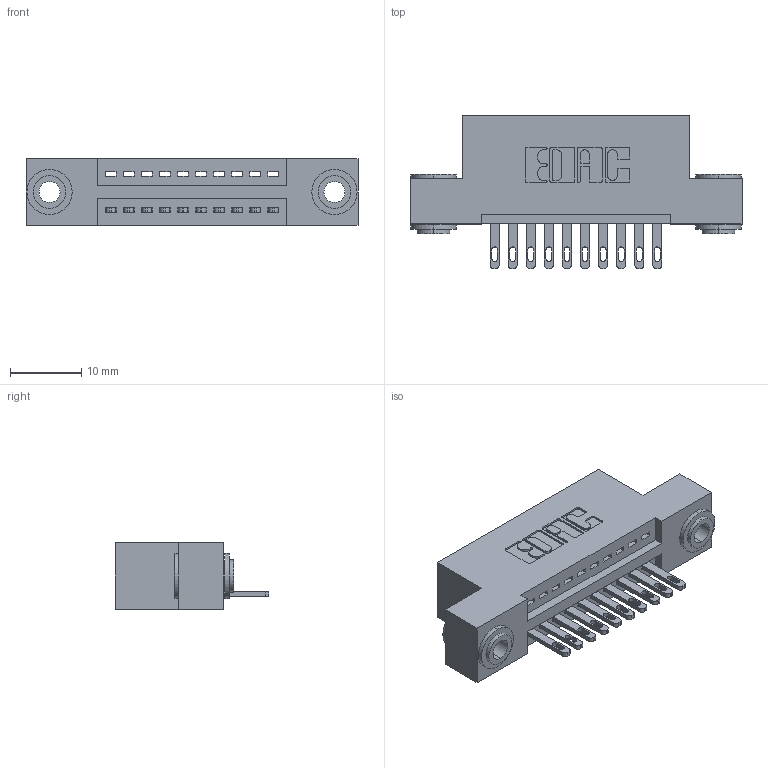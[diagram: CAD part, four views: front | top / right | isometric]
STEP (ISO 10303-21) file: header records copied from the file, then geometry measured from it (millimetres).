
FILE_DESCRIPTION (( 'STEP AP203' ), '1' );
FILE_NAME ('345-010-500-103.STEP', '2019-10-03T21:06:27', ( '' ), ( '' ), 'SwSTEP 2.0', 'SolidWorks 2016', '' );
FILE_SCHEMA (( 'CONFIG_CONTROL_DESIGN' ));
Length unit declared in the file: inch
Products named in the file (4): 345-010-500-103; 345-250-002_345-250-002-102; 345-292-001_345-293-100; 345 Part_Flush Mounting Lugs - 0.156 Dia-TH
Assembly tree (13 placements, depth 2):
  345-010-500-103
    345 Part_Flush Mounting Lugs - 0.156 Dia-TH
    345-292-001_345-293-100  x10
    345-250-002_345-250-002-102  x2
Bounding box: 46.61 x 21.51 x 9.4 mm (x, y, z)
Volume: 4190.4 mm3; surface area: 5370.7 mm2
Topology: 13 solids, 13 shells, 704 faces, 2097 edges, 1394 vertices
Faces by surface type: plane 430, cylinder 266, cone 8
Entity records: 12414 total; most frequent: CARTESIAN_POINT 2129, ORIENTED_EDGE 2066, DIRECTION 1939, EDGE_CURVE 1033, LINE 833, VECTOR 833, VERTEX_POINT 686, AXIS2_PLACEMENT_3D 553
